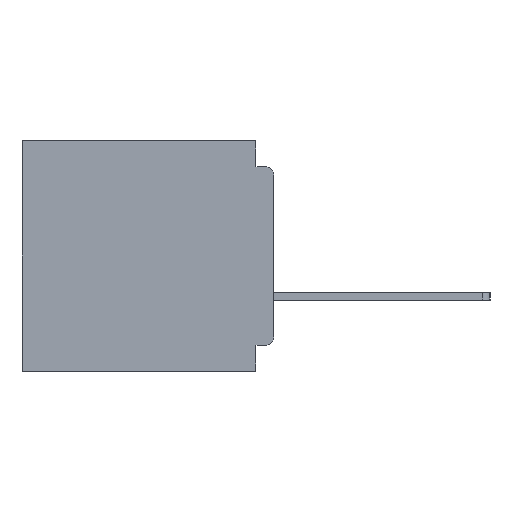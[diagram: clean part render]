
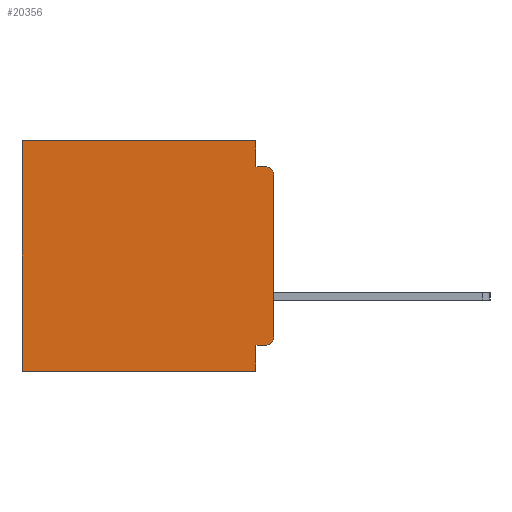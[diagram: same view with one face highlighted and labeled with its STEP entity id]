
A CAD part, left-side view. The second image highlights one B-rep face of the part: STEP entity #20356.
In plain terms, the highlighted planar face has unit normal (-1, 0, 0).
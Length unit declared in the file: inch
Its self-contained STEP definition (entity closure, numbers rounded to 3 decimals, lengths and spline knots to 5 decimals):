
#664 = VERTEX_POINT ( 'NONE', #20215 ) ;
#970 = VERTEX_POINT ( 'NONE', #1604 ) ;
#1517 = VERTEX_POINT ( 'NONE', #17645 ) ;
#1604 = CARTESIAN_POINT ( 'NONE',  ( 0.3, 0.031, 0. ) ) ;
#1751 = DIRECTION ( 'NONE',  ( 0., 0., -1. ) ) ;
#1752 = CARTESIAN_POINT ( 'NONE',  ( 0.3, 0., -0.045 ) ) ;
#1933 = DIRECTION ( 'NONE',  ( 0., 0., -1. ) ) ;
#2230 = VECTOR ( 'NONE', #12101, 39.37008 ) ;
#2842 = CARTESIAN_POINT ( 'NONE',  ( 0.3, 0.437, 0. ) ) ;
#2886 = LINE ( 'NONE', #16283, #32124 ) ;
#3033 = DIRECTION ( 'NONE',  ( 0., 0., -1. ) ) ;
#3399 = ORIENTED_EDGE ( 'NONE', *, *, #21666, .T. ) ;
#3494 = CARTESIAN_POINT ( 'NONE',  ( 0.3, 0.015, -0.06 ) ) ;
#3644 = VECTOR ( 'NONE', #3033, 39.37008 ) ;
#3873 = CARTESIAN_POINT ( 'NONE',  ( 0.3, 0., -0.06 ) ) ;
#3928 = EDGE_CURVE ( 'NONE', #16329, #27241, #26214, .T. ) ;
#3994 = LINE ( 'NONE', #12255, #23974 ) ;
#4465 = CARTESIAN_POINT ( 'NONE',  ( 0.3, 0.031, -0.045 ) ) ;
#5677 = CARTESIAN_POINT ( 'NONE',  ( 0.3, 0., -0.4 ) ) ;
#6700 = VERTEX_POINT ( 'NONE', #4465 ) ;
#6979 = ORIENTED_EDGE ( 'NONE', *, *, #19486, .F. ) ;
#7709 = CARTESIAN_POINT ( 'NONE',  ( 0.3, 0., -0.4 ) ) ;
#7748 = DIRECTION ( 'NONE',  ( 1., 0., 0. ) ) ;
#8350 = VECTOR ( 'NONE', #10886, 39.37008 ) ;
#8664 = AXIS2_PLACEMENT_3D ( 'NONE', #3494, #11474, #1751 ) ;
#8783 = EDGE_CURVE ( 'NONE', #970, #6700, #3994, .T. ) ;
#8824 = VERTEX_POINT ( 'NONE', #32146 ) ;
#8843 = VECTOR ( 'NONE', #16157, 39.37008 ) ;
#9635 = EDGE_CURVE ( 'NONE', #6700, #27241, #31324, .T. ) ;
#10886 = DIRECTION ( 'NONE',  ( 0., 1., 0. ) ) ;
#11474 = DIRECTION ( 'NONE',  ( -1., 0., 0. ) ) ;
#12101 = DIRECTION ( 'NONE',  ( 0., 1., 0. ) ) ;
#12255 = CARTESIAN_POINT ( 'NONE',  ( 0.3, 0.031, 0. ) ) ;
#14794 = EDGE_LOOP ( 'NONE', ( #36548, #15861, #16748, #31716, #3399, #18498, #35294, #6979, #16323, #31270 ) ) ;
#15075 = AXIS2_PLACEMENT_3D ( 'NONE', #33087, #7748, #27529 ) ;
#15662 = CARTESIAN_POINT ( 'NONE',  ( 0.3, 0.015, -0.045 ) ) ;
#15861 = ORIENTED_EDGE ( 'NONE', *, *, #3928, .T. ) ;
#16157 = DIRECTION ( 'NONE',  ( 0., 1., 0. ) ) ;
#16202 = PLANE ( 'NONE',  #15075 ) ;
#16283 = CARTESIAN_POINT ( 'NONE',  ( 0.3, 0.031, -0.4 ) ) ;
#16323 = ORIENTED_EDGE ( 'NONE', *, *, #20106, .F. ) ;
#16329 = VERTEX_POINT ( 'NONE', #3873 ) ;
#16748 = ORIENTED_EDGE ( 'NONE', *, *, #9635, .F. ) ;
#16896 = FACE_OUTER_BOUND ( 'NONE', #14794, .T. ) ;
#17353 = LINE ( 'NONE', #29027, #2230 ) ;
#17453 = CARTESIAN_POINT ( 'NONE',  ( 0.3, 0.031, -0.4 ) ) ;
#17645 = CARTESIAN_POINT ( 'NONE',  ( 0.3, 0.031, -0.355 ) ) ;
#18498 = ORIENTED_EDGE ( 'NONE', *, *, #30730, .T. ) ;
#18934 = DIRECTION ( 'NONE',  ( -1., 0., 0. ) ) ;
#19103 = DIRECTION ( 'NONE',  ( 0., 0., -1. ) ) ;
#19486 = EDGE_CURVE ( 'NONE', #1517, #21912, #2886, .T. ) ;
#19807 = DIRECTION ( 'NONE',  ( 0., 0., -1. ) ) ;
#19987 = EDGE_CURVE ( 'NONE', #664, #8824, #22840, .T. ) ;
#20106 = EDGE_CURVE ( 'NONE', #664, #1517, #17353, .T. ) ;
#20215 = CARTESIAN_POINT ( 'NONE',  ( 0.3, 0.015, -0.355 ) ) ;
#20257 = AXIS2_PLACEMENT_3D ( 'NONE', #35838, #18934, #1933 ) ;
#20356 = ADVANCED_FACE ( 'NONE', ( #16896 ), #16202, .F. ) ;
#20819 = VERTEX_POINT ( 'NONE', #20995 ) ;
#20822 = DIRECTION ( 'NONE',  ( 0., 0., -1. ) ) ;
#20995 = CARTESIAN_POINT ( 'NONE',  ( 0.3, 0.437, -0.4 ) ) ;
#21009 = EDGE_CURVE ( 'NONE', #21912, #20819, #32288, .T. ) ;
#21666 = EDGE_CURVE ( 'NONE', #970, #32851, #30865, .T. ) ;
#21912 = VERTEX_POINT ( 'NONE', #17453 ) ;
#22840 = CIRCLE ( 'NONE', #20257, 0.015 ) ;
#23003 = VECTOR ( 'NONE', #30091, 39.37008 ) ;
#23974 = VECTOR ( 'NONE', #20822, 39.37008 ) ;
#24232 = VECTOR ( 'NONE', #19807, 39.37008 ) ;
#26214 = CIRCLE ( 'NONE', #8664, 0.015 ) ;
#26235 = LINE ( 'NONE', #34090, #3644 ) ;
#27241 = VERTEX_POINT ( 'NONE', #15662 ) ;
#27529 = DIRECTION ( 'NONE',  ( 0., 0., -1. ) ) ;
#29027 = CARTESIAN_POINT ( 'NONE',  ( 0.3, 0., -0.355 ) ) ;
#30091 = DIRECTION ( 'NONE',  ( 0., -1., 0. ) ) ;
#30730 = EDGE_CURVE ( 'NONE', #32851, #20819, #26235, .T. ) ;
#30865 = LINE ( 'NONE', #36209, #8350 ) ;
#31270 = ORIENTED_EDGE ( 'NONE', *, *, #19987, .T. ) ;
#31324 = LINE ( 'NONE', #1752, #23003 ) ;
#31716 = ORIENTED_EDGE ( 'NONE', *, *, #8783, .F. ) ;
#32124 = VECTOR ( 'NONE', #19103, 39.37008 ) ;
#32146 = CARTESIAN_POINT ( 'NONE',  ( 0.3, 0., -0.34 ) ) ;
#32288 = LINE ( 'NONE', #7709, #8843 ) ;
#32586 = LINE ( 'NONE', #5677, #24232 ) ;
#32851 = VERTEX_POINT ( 'NONE', #2842 ) ;
#33087 = CARTESIAN_POINT ( 'NONE',  ( 0.3, 0., -0.4 ) ) ;
#33531 = EDGE_CURVE ( 'NONE', #16329, #8824, #32586, .T. ) ;
#34090 = CARTESIAN_POINT ( 'NONE',  ( 0.3, 0.437, -0.4 ) ) ;
#35294 = ORIENTED_EDGE ( 'NONE', *, *, #21009, .F. ) ;
#35838 = CARTESIAN_POINT ( 'NONE',  ( 0.3, 0.015, -0.34 ) ) ;
#36209 = CARTESIAN_POINT ( 'NONE',  ( 0.3, 0., 0. ) ) ;
#36548 = ORIENTED_EDGE ( 'NONE', *, *, #33531, .F. ) ;
